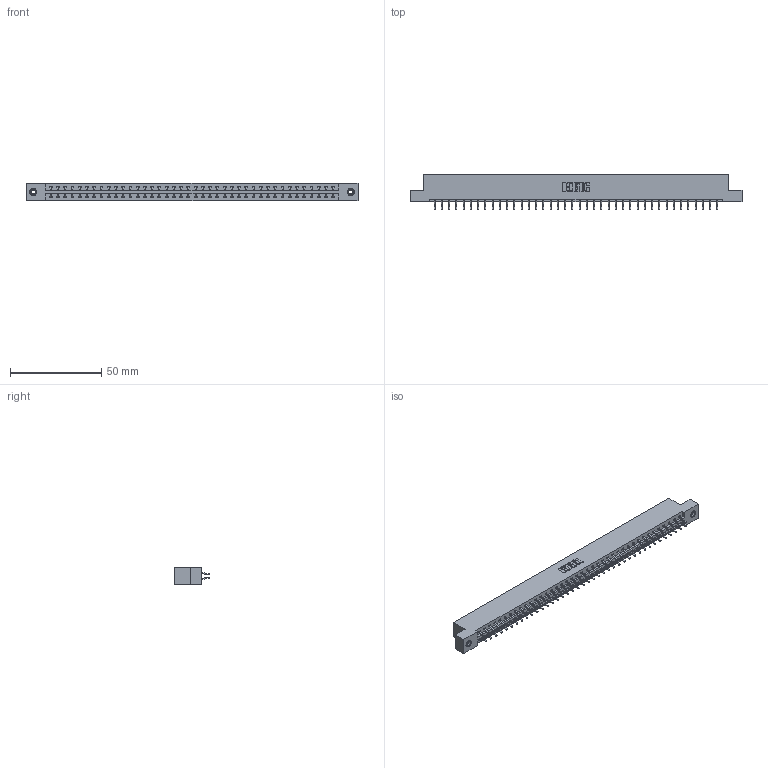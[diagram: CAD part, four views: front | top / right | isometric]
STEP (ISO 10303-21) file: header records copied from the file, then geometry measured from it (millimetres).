
FILE_DESCRIPTION (( 'STEP AP203' ), '1' );
FILE_NAME ('387-080-556-208.STEP', '2019-10-22T22:38:51', ( '' ), ( '' ), 'SwSTEP 2.0', 'SolidWorks 2016', '' );
FILE_SCHEMA (( 'CONFIG_CONTROL_DESIGN' ));
Length unit declared in the file: inch
Products named in the file (4): 387-080-556-208; 337 Part_Flush Mounting Lugs - 0.156 Dia-TI; 345-292-001_556 Tail; 345-250-001_345-250-003-102
Assembly tree (83 placements, depth 2):
  387-080-556-208
    337 Part_Flush Mounting Lugs - 0.156 Dia-TI
    345-292-001_556 Tail  x80
    345-250-001_345-250-003-102  x2
Bounding box: 181.51 x 19.57 x 9.4 mm (x, y, z)
Volume: 19092.5 mm3; surface area: 21504.2 mm2
Topology: 83 solids, 83 shells, 4974 faces, 14767 edges, 9730 vertices
Faces by surface type: plane 3462, cylinder 1496, cone 12, torus 4
Entity records: 32678 total; most frequent: CARTESIAN_POINT 5501, ORIENTED_EDGE 5418, DIRECTION 4703, EDGE_CURVE 2709, VECTOR 2553, LINE 2553, VERTEX_POINT 1800, AXIS2_PLACEMENT_3D 1075
